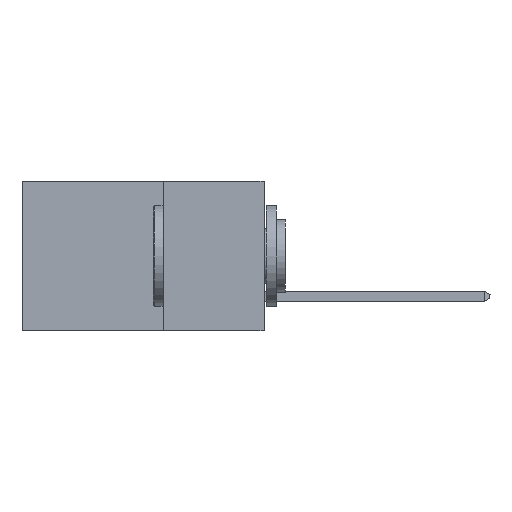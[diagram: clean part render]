
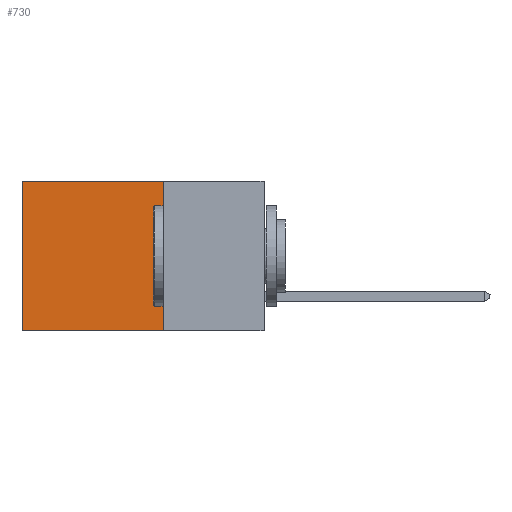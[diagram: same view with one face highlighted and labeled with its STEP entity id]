
A CAD part, left-side view. The second image highlights one B-rep face of the part: STEP entity #730.
In plain terms, the highlighted planar face has unit normal (-1, 0, 0).
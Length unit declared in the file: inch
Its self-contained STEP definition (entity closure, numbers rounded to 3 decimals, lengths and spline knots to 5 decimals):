
#133 = CARTESIAN_POINT ( 'NONE',  ( 0.2615, 0.6, -0.37 ) ) ;
#730 = ADVANCED_FACE ( 'NONE', ( #6568 ), #18521, .F. ) ;
#1193 = CARTESIAN_POINT ( 'NONE',  ( 0.2615, 0.25, -0.37 ) ) ;
#2719 = DIRECTION ( 'NONE',  ( 0., 0., -1. ) ) ;
#2989 = DIRECTION ( 'NONE',  ( 0., 1., 0. ) ) ;
#4090 = CARTESIAN_POINT ( 'NONE',  ( 0.2615, 0.6, -0.37 ) ) ;
#4914 = LINE ( 'NONE', #1193, #11809 ) ;
#5295 = EDGE_CURVE ( 'NONE', #17483, #13123, #9875, .T. ) ;
#6444 = DIRECTION ( 'NONE',  ( 1., 0., 0. ) ) ;
#6568 = FACE_OUTER_BOUND ( 'NONE', #7644, .T. ) ;
#6604 = VECTOR ( 'NONE', #11564, 39.37008 ) ;
#6909 = LINE ( 'NONE', #8730, #16899 ) ;
#6986 = AXIS2_PLACEMENT_3D ( 'NONE', #22651, #6444, #2719 ) ;
#7012 = CARTESIAN_POINT ( 'NONE',  ( 0.2615, 0.6, 0. ) ) ;
#7644 = EDGE_LOOP ( 'NONE', ( #19032, #20850, #11343, #24598 ) ) ;
#8655 = EDGE_CURVE ( 'NONE', #12130, #13123, #4914, .T. ) ;
#8730 = CARTESIAN_POINT ( 'NONE',  ( 0.2615, 0.25, -0.37 ) ) ;
#9875 = LINE ( 'NONE', #4090, #22100 ) ;
#11343 = ORIENTED_EDGE ( 'NONE', *, *, #17910, .F. ) ;
#11564 = DIRECTION ( 'NONE',  ( 0., 1., 0. ) ) ;
#11809 = VECTOR ( 'NONE', #2989, 39.37008 ) ;
#11823 = VERTEX_POINT ( 'NONE', #19716 ) ;
#12130 = VERTEX_POINT ( 'NONE', #17022 ) ;
#13123 = VERTEX_POINT ( 'NONE', #133 ) ;
#14501 = DIRECTION ( 'NONE',  ( 0., 0., -1. ) ) ;
#15178 = LINE ( 'NONE', #19165, #6604 ) ;
#16037 = DIRECTION ( 'NONE',  ( 0., 0., -1. ) ) ;
#16827 = EDGE_CURVE ( 'NONE', #11823, #17483, #15178, .T. ) ;
#16899 = VECTOR ( 'NONE', #14501, 39.37008 ) ;
#17022 = CARTESIAN_POINT ( 'NONE',  ( 0.2615, 0.25, -0.37 ) ) ;
#17483 = VERTEX_POINT ( 'NONE', #7012 ) ;
#17910 = EDGE_CURVE ( 'NONE', #11823, #12130, #6909, .T. ) ;
#18521 = PLANE ( 'NONE',  #6986 ) ;
#19032 = ORIENTED_EDGE ( 'NONE', *, *, #5295, .T. ) ;
#19165 = CARTESIAN_POINT ( 'NONE',  ( 0.2615, 0.25, 0. ) ) ;
#19716 = CARTESIAN_POINT ( 'NONE',  ( 0.2615, 0.25, 0. ) ) ;
#20850 = ORIENTED_EDGE ( 'NONE', *, *, #8655, .F. ) ;
#22100 = VECTOR ( 'NONE', #16037, 39.37008 ) ;
#22651 = CARTESIAN_POINT ( 'NONE',  ( 0.2615, 0.25, -0.37 ) ) ;
#24598 = ORIENTED_EDGE ( 'NONE', *, *, #16827, .T. ) ;
